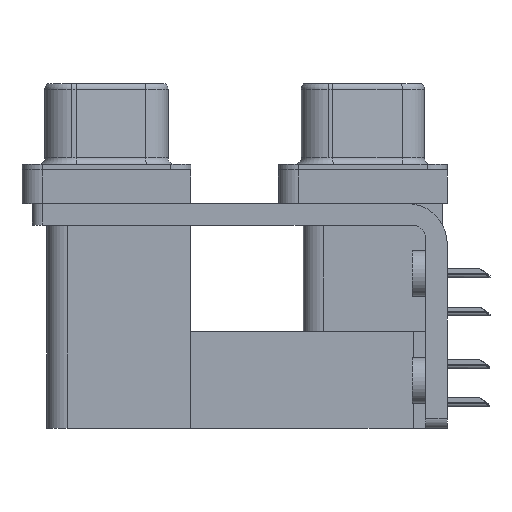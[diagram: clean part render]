
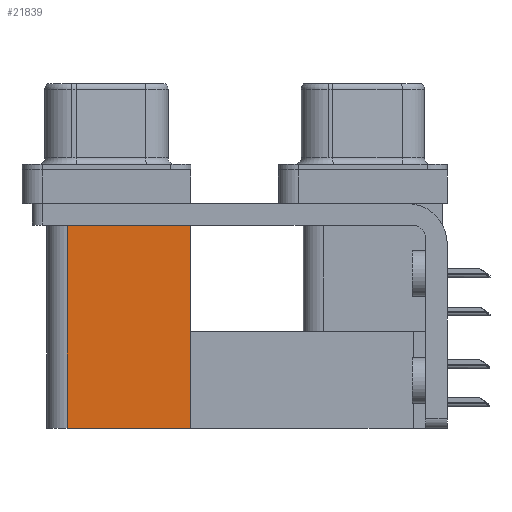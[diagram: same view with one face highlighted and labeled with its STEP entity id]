
A CAD part, left-side view. The second image highlights one B-rep face of the part: STEP entity #21839.
In plain terms, the highlighted planar face has unit normal (-1, 0, 0).
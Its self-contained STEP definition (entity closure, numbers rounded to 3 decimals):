
#101 = CARTESIAN_POINT ( 'NONE',  ( 3.7, 12.775, -19.2 ) ) ;
#938 = LINE ( 'NONE', #101, #20694 ) ;
#1151 = EDGE_CURVE ( 'NONE', #8939, #14083, #938, .T. ) ;
#2106 = DIRECTION ( 'NONE',  ( 0., 1., 0. ) ) ;
#2743 = AXIS2_PLACEMENT_3D ( 'NONE', #23845, #11468, #24695 ) ;
#3872 = DIRECTION ( 'NONE',  ( 0., 0., 1. ) ) ;
#4139 = PLANE ( 'NONE',  #2743 ) ;
#7947 = ORIENTED_EDGE ( 'NONE', *, *, #10854, .F. ) ;
#8939 = VERTEX_POINT ( 'NONE', #36969 ) ;
#9172 = EDGE_CURVE ( 'NONE', #14083, #37013, #35440, .T. ) ;
#10854 = EDGE_CURVE ( 'NONE', #40759, #37013, #23388, .T. ) ;
#11055 = FACE_OUTER_BOUND ( 'NONE', #38732, .T. ) ;
#11468 = DIRECTION ( 'NONE',  ( 1., 0., 0. ) ) ;
#14083 = VERTEX_POINT ( 'NONE', #34868 ) ;
#18932 = ORIENTED_EDGE ( 'NONE', *, *, #1151, .T. ) ;
#20694 = VECTOR ( 'NONE', #23281, 1000. ) ;
#21839 = ADVANCED_FACE ( 'NONE', ( #11055 ), #4139, .F. ) ;
#21977 = ORIENTED_EDGE ( 'NONE', *, *, #23489, .F. ) ;
#23281 = DIRECTION ( 'NONE',  ( 0., 0., 1. ) ) ;
#23388 = LINE ( 'NONE', #33328, #41964 ) ;
#23489 = EDGE_CURVE ( 'NONE', #8939, #40759, #41745, .T. ) ;
#23845 = CARTESIAN_POINT ( 'NONE',  ( 3.7, 12.775, -19.2 ) ) ;
#23858 = CARTESIAN_POINT ( 'NONE',  ( 3.7, 21.975, -19.2 ) ) ;
#24695 = DIRECTION ( 'NONE',  ( 0., 0., -1. ) ) ;
#26789 = VECTOR ( 'NONE', #2106, 1000. ) ;
#28343 = CARTESIAN_POINT ( 'NONE',  ( 3.7, 12.775, -19.2 ) ) ;
#33207 = ORIENTED_EDGE ( 'NONE', *, *, #9172, .T. ) ;
#33328 = CARTESIAN_POINT ( 'NONE',  ( 3.7, 21.975, -19.2 ) ) ;
#33733 = VECTOR ( 'NONE', #34391, 1000. ) ;
#34391 = DIRECTION ( 'NONE',  ( 0., 1., 0. ) ) ;
#34868 = CARTESIAN_POINT ( 'NONE',  ( 3.7, 12.775, -2.5 ) ) ;
#35440 = LINE ( 'NONE', #41287, #26789 ) ;
#35720 = CARTESIAN_POINT ( 'NONE',  ( 3.7, 21.975, -2.5 ) ) ;
#36969 = CARTESIAN_POINT ( 'NONE',  ( 3.7, 12.775, -19.2 ) ) ;
#37013 = VERTEX_POINT ( 'NONE', #35720 ) ;
#38732 = EDGE_LOOP ( 'NONE', ( #33207, #7947, #21977, #18932 ) ) ;
#40759 = VERTEX_POINT ( 'NONE', #23858 ) ;
#41287 = CARTESIAN_POINT ( 'NONE',  ( 3.7, 12.775, -2.5 ) ) ;
#41745 = LINE ( 'NONE', #28343, #33733 ) ;
#41964 = VECTOR ( 'NONE', #3872, 1000. ) ;
